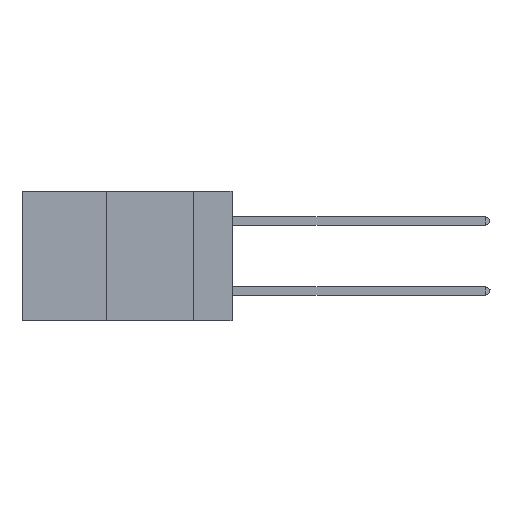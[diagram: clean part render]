
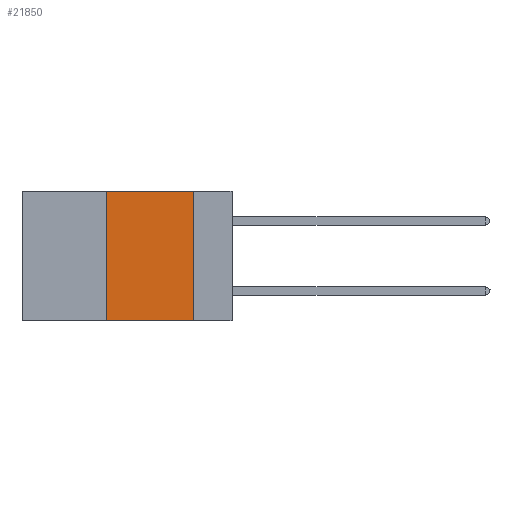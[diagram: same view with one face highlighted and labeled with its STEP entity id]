
A CAD part, left-side view. The second image highlights one B-rep face of the part: STEP entity #21850.
In plain terms, the highlighted planar face has unit normal (-1, 0, 0).
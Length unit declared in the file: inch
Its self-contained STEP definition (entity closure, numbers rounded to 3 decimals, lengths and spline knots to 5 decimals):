
#357 = ORIENTED_EDGE ( 'NONE', *, *, #19748, .F. ) ;
#807 = DIRECTION ( 'NONE',  ( 0., 0., 1. ) ) ;
#1182 = PLANE ( 'NONE',  #18176 ) ;
#2201 = LINE ( 'NONE', #7808, #5461 ) ;
#2463 = CARTESIAN_POINT ( 'NONE',  ( 0., 0.11, -0.37 ) ) ;
#3175 = VERTEX_POINT ( 'NONE', #2463 ) ;
#4146 = DIRECTION ( 'NONE',  ( 0., -1., 0. ) ) ;
#4227 = VERTEX_POINT ( 'NONE', #18780 ) ;
#4495 = EDGE_CURVE ( 'NONE', #22354, #3175, #22824, .T. ) ;
#4952 = DIRECTION ( 'NONE',  ( 0., 0., -1. ) ) ;
#5143 = DIRECTION ( 'NONE',  ( 0., -1., 0. ) ) ;
#5461 = VECTOR ( 'NONE', #4146, 39.37008 ) ;
#6411 = ORIENTED_EDGE ( 'NONE', *, *, #4495, .F. ) ;
#6724 = ORIENTED_EDGE ( 'NONE', *, *, #14240, .F. ) ;
#6841 = CARTESIAN_POINT ( 'NONE',  ( 0., 0.6, -0.37 ) ) ;
#7736 = ORIENTED_EDGE ( 'NONE', *, *, #11123, .T. ) ;
#7808 = CARTESIAN_POINT ( 'NONE',  ( 0., 0.6, 0. ) ) ;
#9800 = FACE_OUTER_BOUND ( 'NONE', #16751, .T. ) ;
#10189 = CARTESIAN_POINT ( 'NONE',  ( 0., 0.11, 0. ) ) ;
#11123 = EDGE_CURVE ( 'NONE', #13705, #3175, #18052, .T. ) ;
#11628 = VECTOR ( 'NONE', #807, 39.37008 ) ;
#12226 = LINE ( 'NONE', #14161, #11628 ) ;
#12878 = DIRECTION ( 'NONE',  ( 0., 0., -1. ) ) ;
#13705 = VERTEX_POINT ( 'NONE', #14183 ) ;
#14161 = CARTESIAN_POINT ( 'NONE',  ( 0., 0.36, 0. ) ) ;
#14183 = CARTESIAN_POINT ( 'NONE',  ( 0., 0.36, -0.37 ) ) ;
#14212 = CARTESIAN_POINT ( 'NONE',  ( 0., 0.6, 0. ) ) ;
#14240 = EDGE_CURVE ( 'NONE', #13705, #4227, #12226, .T. ) ;
#16066 = DIRECTION ( 'NONE',  ( 1., 0., 0. ) ) ;
#16751 = EDGE_LOOP ( 'NONE', ( #6411, #357, #6724, #7736 ) ) ;
#18052 = LINE ( 'NONE', #6841, #21358 ) ;
#18176 = AXIS2_PLACEMENT_3D ( 'NONE', #14212, #16066, #4952 ) ;
#18780 = CARTESIAN_POINT ( 'NONE',  ( 0., 0.36, 0. ) ) ;
#19748 = EDGE_CURVE ( 'NONE', #4227, #22354, #2201, .T. ) ;
#21358 = VECTOR ( 'NONE', #5143, 39.37008 ) ;
#21619 = CARTESIAN_POINT ( 'NONE',  ( 0., 0.11, 0. ) ) ;
#21850 = ADVANCED_FACE ( 'NONE', ( #9800 ), #1182, .F. ) ;
#22354 = VERTEX_POINT ( 'NONE', #21619 ) ;
#22824 = LINE ( 'NONE', #10189, #23430 ) ;
#23430 = VECTOR ( 'NONE', #12878, 39.37008 ) ;
